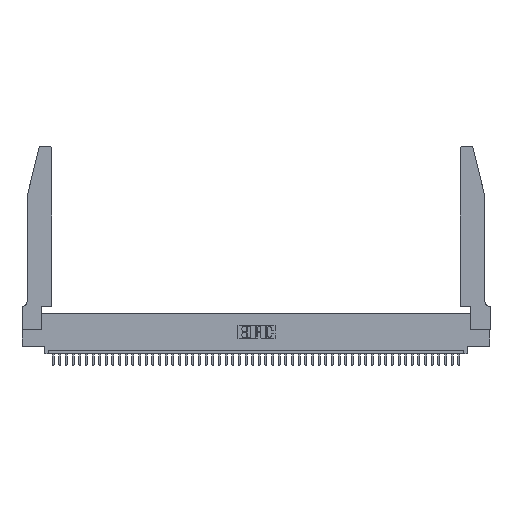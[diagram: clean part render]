
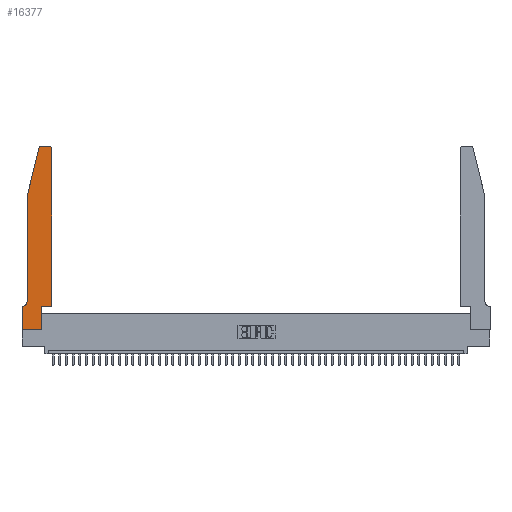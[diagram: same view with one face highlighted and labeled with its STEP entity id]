
A CAD part, top view. The second image highlights one B-rep face of the part: STEP entity #16377.
In plain terms, the highlighted planar face has unit normal (0, 0, 1).
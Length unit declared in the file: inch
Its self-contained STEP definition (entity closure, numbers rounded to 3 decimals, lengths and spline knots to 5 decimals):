
#1022 = AXIS2_PLACEMENT_3D ( 'NONE', #48002, #44725, #6861 ) ;
#1431 = EDGE_CURVE ( 'NONE', #22276, #22814, #48622, .T. ) ;
#1476 = VERTEX_POINT ( 'NONE', #28309 ) ;
#1901 = VERTEX_POINT ( 'NONE', #28737 ) ;
#2796 = LINE ( 'NONE', #32217, #35388 ) ;
#2850 = EDGE_CURVE ( 'NONE', #30736, #22276, #44938, .T. ) ;
#2923 = ORIENTED_EDGE ( 'NONE', *, *, #37841, .T. ) ;
#4275 = VECTOR ( 'NONE', #27410, 39.37008 ) ;
#4560 = ORIENTED_EDGE ( 'NONE', *, *, #18495, .T. ) ;
#5455 = DIRECTION ( 'NONE',  ( -1., 0., 0. ) ) ;
#5926 = CARTESIAN_POINT ( 'NONE',  ( 0.0755, 0.42, 0.37 ) ) ;
#6332 = LINE ( 'NONE', #28282, #43005 ) ;
#6341 = EDGE_CURVE ( 'NONE', #43518, #1476, #18671, .T. ) ;
#6563 = ORIENTED_EDGE ( 'NONE', *, *, #19594, .T. ) ;
#6861 = DIRECTION ( 'NONE',  ( -1., 0., 0. ) ) ;
#7251 = CARTESIAN_POINT ( 'NONE',  ( 0.2865, 0.35, 0.37 ) ) ;
#7851 = EDGE_CURVE ( 'NONE', #22814, #43518, #44418, .T. ) ;
#9195 = DIRECTION ( 'NONE',  ( 1., 0., 0. ) ) ;
#9589 = ORIENTED_EDGE ( 'NONE', *, *, #2850, .T. ) ;
#10172 = LINE ( 'NONE', #7251, #17322 ) ;
#10508 = CARTESIAN_POINT ( 'NONE',  ( 0.2865, 0., 0.37 ) ) ;
#11909 = CARTESIAN_POINT ( 'NONE',  ( 0.0755, 2., 0.37 ) ) ;
#14271 = EDGE_CURVE ( 'NONE', #41152, #16282, #36138, .T. ) ;
#15573 = ORIENTED_EDGE ( 'NONE', *, *, #6341, .T. ) ;
#15953 = VECTOR ( 'NONE', #5455, 39.37008 ) ;
#16235 = DIRECTION ( 'NONE',  ( 1., 0., 0. ) ) ;
#16282 = VERTEX_POINT ( 'NONE', #10508 ) ;
#16377 = ADVANCED_FACE ( 'NONE', ( #36580 ), #41252, .T. ) ;
#16580 = CARTESIAN_POINT ( 'NONE',  ( 0.0755, 0.35, 0.37 ) ) ;
#16637 = EDGE_CURVE ( 'NONE', #17645, #33696, #6332, .T. ) ;
#17257 = DIRECTION ( 'NONE',  ( 0., -1., 0. ) ) ;
#17322 = VECTOR ( 'NONE', #22192, 39.37008 ) ;
#17645 = VERTEX_POINT ( 'NONE', #42551 ) ;
#18367 = DIRECTION ( 'NONE',  ( 0., -1., 0. ) ) ;
#18397 = VECTOR ( 'NONE', #21619, 39.37008 ) ;
#18495 = EDGE_CURVE ( 'NONE', #34262, #30736, #29833, .T. ) ;
#18671 = CIRCLE ( 'NONE', #1022, 0.07 ) ;
#18677 = CARTESIAN_POINT ( 'NONE',  ( 0.0755, 2., 0.37 ) ) ;
#19594 = EDGE_CURVE ( 'NONE', #16282, #24246, #10172, .T. ) ;
#20091 = LINE ( 'NONE', #16580, #15953 ) ;
#20722 = CARTESIAN_POINT ( 'NONE',  ( 0., 0., 0.37 ) ) ;
#20778 = ORIENTED_EDGE ( 'NONE', *, *, #1431, .T. ) ;
#21379 = AXIS2_PLACEMENT_3D ( 'NONE', #26116, #34056, #45084 ) ;
#21619 = DIRECTION ( 'NONE',  ( 1., 0., 0. ) ) ;
#21704 = CARTESIAN_POINT ( 'NONE',  ( 0.2605, 2.75, 0.37 ) ) ;
#22192 = DIRECTION ( 'NONE',  ( 0., 1., 0. ) ) ;
#22276 = VERTEX_POINT ( 'NONE', #36570 ) ;
#22814 = VERTEX_POINT ( 'NONE', #43100 ) ;
#23054 = CARTESIAN_POINT ( 'NONE',  ( 0.284, 2.75, 0.37 ) ) ;
#23545 = DIRECTION ( 'NONE',  ( 0., 0., 1. ) ) ;
#23699 = CARTESIAN_POINT ( 'NONE',  ( 0.4205, 2.72, 0.37 ) ) ;
#24246 = VERTEX_POINT ( 'NONE', #43480 ) ;
#25144 = ORIENTED_EDGE ( 'NONE', *, *, #35989, .T. ) ;
#25907 = DIRECTION ( 'NONE',  ( 1., 0., 0. ) ) ;
#26116 = CARTESIAN_POINT ( 'NONE',  ( 0.284, 2.72, 0.37 ) ) ;
#26746 = AXIS2_PLACEMENT_3D ( 'NONE', #30321, #37340, #25907 ) ;
#27410 = DIRECTION ( 'NONE',  ( -1., 0., 0. ) ) ;
#28149 = CARTESIAN_POINT ( 'NONE',  ( 0., 0., 0.37 ) ) ;
#28282 = CARTESIAN_POINT ( 'NONE',  ( 0.4505, 0.35, 0.37 ) ) ;
#28309 = CARTESIAN_POINT ( 'NONE',  ( 0.0055, 0.35, 0.37 ) ) ;
#28737 = CARTESIAN_POINT ( 'NONE',  ( 0., 0.35, 0.37 ) ) ;
#28838 = EDGE_LOOP ( 'NONE', ( #4560, #9589, #20778, #32004, #15573, #48659, #2923, #38400, #6563, #36614, #48434, #25144 ) ) ;
#29786 = AXIS2_PLACEMENT_3D ( 'NONE', #23699, #23545, #16235 ) ;
#29833 = LINE ( 'NONE', #21704, #4275 ) ;
#30321 = CARTESIAN_POINT ( 'NONE',  ( 0., 0.35, 0.37 ) ) ;
#30736 = VERTEX_POINT ( 'NONE', #23054 ) ;
#31579 = DIRECTION ( 'NONE',  ( 0., 1., 0. ) ) ;
#32004 = ORIENTED_EDGE ( 'NONE', *, *, #7851, .T. ) ;
#32061 = VECTOR ( 'NONE', #17257, 39.37008 ) ;
#32217 = CARTESIAN_POINT ( 'NONE',  ( 0.4505, 0.35, 0.37 ) ) ;
#33696 = VERTEX_POINT ( 'NONE', #46148 ) ;
#34056 = DIRECTION ( 'NONE',  ( 0., 0., 1. ) ) ;
#34262 = VERTEX_POINT ( 'NONE', #45948 ) ;
#34382 = VECTOR ( 'NONE', #18367, 39.37008 ) ;
#35388 = VECTOR ( 'NONE', #9195, 39.37008 ) ;
#35989 = EDGE_CURVE ( 'NONE', #33696, #34262, #48180, .T. ) ;
#36138 = LINE ( 'NONE', #41240, #18397 ) ;
#36570 = CARTESIAN_POINT ( 'NONE',  ( 0.25487, 2.72718, 0.37 ) ) ;
#36580 = FACE_OUTER_BOUND ( 'NONE', #28838, .T. ) ;
#36614 = ORIENTED_EDGE ( 'NONE', *, *, #48713, .T. ) ;
#37340 = DIRECTION ( 'NONE',  ( 0., 0., 1. ) ) ;
#37841 = EDGE_CURVE ( 'NONE', #1901, #41152, #48000, .T. ) ;
#38400 = ORIENTED_EDGE ( 'NONE', *, *, #14271, .T. ) ;
#41152 = VERTEX_POINT ( 'NONE', #28149 ) ;
#41213 = EDGE_CURVE ( 'NONE', #1476, #1901, #20091, .T. ) ;
#41240 = CARTESIAN_POINT ( 'NONE',  ( 0., 0., 0.37 ) ) ;
#41252 = PLANE ( 'NONE',  #26746 ) ;
#41547 = VECTOR ( 'NONE', #42678, 39.37008 ) ;
#42551 = CARTESIAN_POINT ( 'NONE',  ( 0.4505, 0.35, 0.37 ) ) ;
#42678 = DIRECTION ( 'NONE',  ( -0.239, -0.971, 0. ) ) ;
#43005 = VECTOR ( 'NONE', #31579, 39.37008 ) ;
#43100 = CARTESIAN_POINT ( 'NONE',  ( 0.0755, 2., 0.37 ) ) ;
#43480 = CARTESIAN_POINT ( 'NONE',  ( 0.2865, 0.35, 0.37 ) ) ;
#43518 = VERTEX_POINT ( 'NONE', #5926 ) ;
#44418 = LINE ( 'NONE', #18677, #34382 ) ;
#44725 = DIRECTION ( 'NONE',  ( 0., 0., -1. ) ) ;
#44938 = CIRCLE ( 'NONE', #21379, 0.03 ) ;
#45084 = DIRECTION ( 'NONE',  ( 1., 0., 0. ) ) ;
#45948 = CARTESIAN_POINT ( 'NONE',  ( 0.4205, 2.75, 0.37 ) ) ;
#46148 = CARTESIAN_POINT ( 'NONE',  ( 0.4505, 2.72, 0.37 ) ) ;
#48000 = LINE ( 'NONE', #20722, #32061 ) ;
#48002 = CARTESIAN_POINT ( 'NONE',  ( 0.0055, 0.42, 0.37 ) ) ;
#48180 = CIRCLE ( 'NONE', #29786, 0.03 ) ;
#48434 = ORIENTED_EDGE ( 'NONE', *, *, #16637, .T. ) ;
#48622 = LINE ( 'NONE', #11909, #41547 ) ;
#48659 = ORIENTED_EDGE ( 'NONE', *, *, #41213, .T. ) ;
#48713 = EDGE_CURVE ( 'NONE', #24246, #17645, #2796, .T. ) ;
